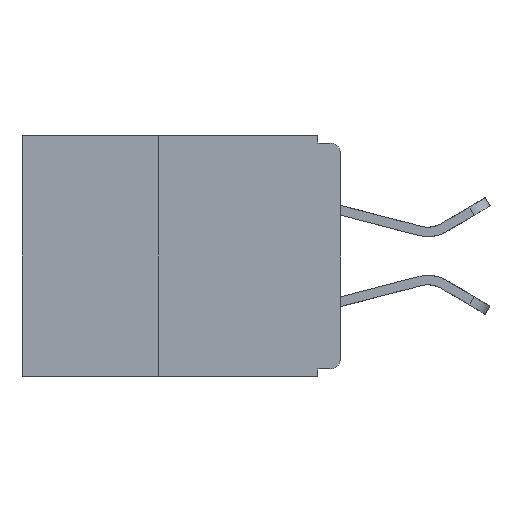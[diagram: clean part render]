
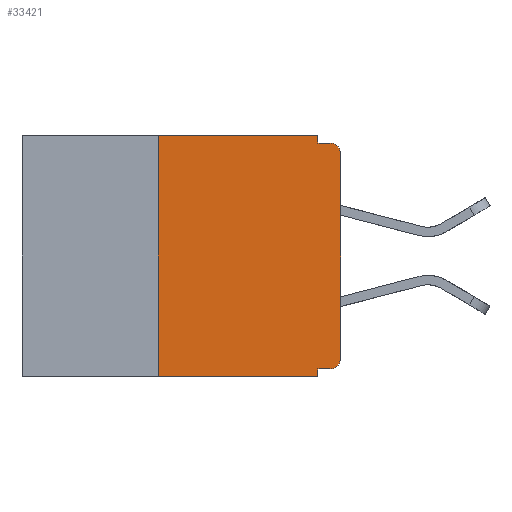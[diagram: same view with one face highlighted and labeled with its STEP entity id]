
A CAD part, left-side view. The second image highlights one B-rep face of the part: STEP entity #33421.
In plain terms, the highlighted planar face has unit normal (-1, 0, 0).
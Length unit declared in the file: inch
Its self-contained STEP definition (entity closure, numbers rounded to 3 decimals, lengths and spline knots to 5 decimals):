
#557 = DIRECTION ( 'NONE',  ( -1., 0., 0. ) ) ;
#912 = VECTOR ( 'NONE', #31816, 39.37008 ) ;
#1109 = DIRECTION ( 'NONE',  ( 0., 0., -1. ) ) ;
#1717 = CARTESIAN_POINT ( 'NONE',  ( 0., 0.031, -0.33 ) ) ;
#2532 = CARTESIAN_POINT ( 'NONE',  ( 0., 0.031, 0. ) ) ;
#2622 = EDGE_CURVE ( 'NONE', #32373, #4309, #14966, .T. ) ;
#2634 = CARTESIAN_POINT ( 'NONE',  ( 0., 0., -0.305 ) ) ;
#3227 = ORIENTED_EDGE ( 'NONE', *, *, #11046, .F. ) ;
#3566 = DIRECTION ( 'NONE',  ( -1., 0., 0. ) ) ;
#3796 = VERTEX_POINT ( 'NONE', #2532 ) ;
#4309 = VERTEX_POINT ( 'NONE', #1717 ) ;
#6083 = DIRECTION ( 'NONE',  ( 0., 0., -1. ) ) ;
#6546 = VERTEX_POINT ( 'NONE', #23697 ) ;
#7873 = VERTEX_POINT ( 'NONE', #2634 ) ;
#8239 = CARTESIAN_POINT ( 'NONE',  ( 0., 0., 0. ) ) ;
#9214 = DIRECTION ( 'NONE',  ( 1., 0., 0. ) ) ;
#9458 = AXIS2_PLACEMENT_3D ( 'NONE', #19245, #3566, #21910 ) ;
#9870 = LINE ( 'NONE', #29517, #32425 ) ;
#10485 = DIRECTION ( 'NONE',  ( 0., 0., 1. ) ) ;
#11046 = EDGE_CURVE ( 'NONE', #21604, #4309, #32266, .T. ) ;
#11399 = CARTESIAN_POINT ( 'NONE',  ( 0., 0.031, -0.33 ) ) ;
#11417 = CARTESIAN_POINT ( 'NONE',  ( 0., 0.031, -0.32 ) ) ;
#11556 = CARTESIAN_POINT ( 'NONE',  ( 0., 0.437, 0. ) ) ;
#11889 = ORIENTED_EDGE ( 'NONE', *, *, #33866, .F. ) ;
#12081 = AXIS2_PLACEMENT_3D ( 'NONE', #16334, #557, #18958 ) ;
#12883 = VERTEX_POINT ( 'NONE', #18671 ) ;
#13077 = CARTESIAN_POINT ( 'NONE',  ( 0., 0., -0.01 ) ) ;
#13196 = DIRECTION ( 'NONE',  ( 0., -1., 0. ) ) ;
#14277 = DIRECTION ( 'NONE',  ( 0., -1., 0. ) ) ;
#14318 = ORIENTED_EDGE ( 'NONE', *, *, #22124, .T. ) ;
#14966 = LINE ( 'NONE', #25424, #912 ) ;
#15114 = ORIENTED_EDGE ( 'NONE', *, *, #20731, .F. ) ;
#15219 = VERTEX_POINT ( 'NONE', #23155 ) ;
#16013 = VECTOR ( 'NONE', #14277, 39.37008 ) ;
#16090 = DIRECTION ( 'NONE',  ( 0., 0., 1. ) ) ;
#16334 = CARTESIAN_POINT ( 'NONE',  ( 0., 0.015, -0.025 ) ) ;
#16618 = CARTESIAN_POINT ( 'NONE',  ( 0., 0.25, 0. ) ) ;
#16709 = ORIENTED_EDGE ( 'NONE', *, *, #23192, .F. ) ;
#16944 = PLANE ( 'NONE',  #30615 ) ;
#17109 = VERTEX_POINT ( 'NONE', #16618 ) ;
#17539 = ORIENTED_EDGE ( 'NONE', *, *, #25066, .F. ) ;
#18671 = CARTESIAN_POINT ( 'NONE',  ( 0., 0.015, -0.01 ) ) ;
#18958 = DIRECTION ( 'NONE',  ( 0., 0., -1. ) ) ;
#19245 = CARTESIAN_POINT ( 'NONE',  ( 0., 0.015, -0.305 ) ) ;
#19425 = VECTOR ( 'NONE', #1109, 39.37008 ) ;
#20249 = LINE ( 'NONE', #32608, #19425 ) ;
#20731 = EDGE_CURVE ( 'NONE', #27944, #12883, #32709, .T. ) ;
#20837 = EDGE_CURVE ( 'NONE', #15219, #12883, #22433, .T. ) ;
#21604 = VERTEX_POINT ( 'NONE', #11417 ) ;
#21910 = DIRECTION ( 'NONE',  ( 0., 0., -1. ) ) ;
#22124 = EDGE_CURVE ( 'NONE', #6546, #7873, #25335, .T. ) ;
#22433 = CIRCLE ( 'NONE', #12081, 0.015 ) ;
#23030 = CARTESIAN_POINT ( 'NONE',  ( 0., 0.25, -0.33 ) ) ;
#23155 = CARTESIAN_POINT ( 'NONE',  ( 0., 0., -0.025 ) ) ;
#23192 = EDGE_CURVE ( 'NONE', #3796, #27944, #20249, .T. ) ;
#23697 = CARTESIAN_POINT ( 'NONE',  ( 0., 0.015, -0.32 ) ) ;
#24935 = CARTESIAN_POINT ( 'NONE',  ( 0., 0.437, 0. ) ) ;
#25066 = EDGE_CURVE ( 'NONE', #17109, #3796, #30035, .T. ) ;
#25335 = CIRCLE ( 'NONE', #9458, 0.015 ) ;
#25423 = ORIENTED_EDGE ( 'NONE', *, *, #33110, .F. ) ;
#25424 = CARTESIAN_POINT ( 'NONE',  ( 0., 0.437, -0.33 ) ) ;
#25801 = VECTOR ( 'NONE', #13196, 39.37008 ) ;
#26629 = ORIENTED_EDGE ( 'NONE', *, *, #29380, .T. ) ;
#27131 = LINE ( 'NONE', #31520, #32418 ) ;
#27588 = DIRECTION ( 'NONE',  ( 0., 0., -1. ) ) ;
#27944 = VERTEX_POINT ( 'NONE', #29426 ) ;
#28269 = ORIENTED_EDGE ( 'NONE', *, *, #20837, .T. ) ;
#29380 = EDGE_CURVE ( 'NONE', #7873, #15219, #33612, .T. ) ;
#29426 = CARTESIAN_POINT ( 'NONE',  ( 0., 0.031, -0.01 ) ) ;
#29517 = CARTESIAN_POINT ( 'NONE',  ( 0., 0., -0.32 ) ) ;
#29577 = FACE_OUTER_BOUND ( 'NONE', #33603, .T. ) ;
#30035 = LINE ( 'NONE', #11556, #16013 ) ;
#30615 = AXIS2_PLACEMENT_3D ( 'NONE', #24935, #9214, #27588 ) ;
#31486 = VECTOR ( 'NONE', #6083, 39.37008 ) ;
#31520 = CARTESIAN_POINT ( 'NONE',  ( 0., 0.25, -0.33 ) ) ;
#31816 = DIRECTION ( 'NONE',  ( 0., -1., 0. ) ) ;
#32112 = DIRECTION ( 'NONE',  ( 0., 1., 0. ) ) ;
#32266 = LINE ( 'NONE', #11399, #31486 ) ;
#32373 = VERTEX_POINT ( 'NONE', #23030 ) ;
#32418 = VECTOR ( 'NONE', #10485, 39.37008 ) ;
#32425 = VECTOR ( 'NONE', #32112, 39.37008 ) ;
#32608 = CARTESIAN_POINT ( 'NONE',  ( 0., 0.031, 0. ) ) ;
#32709 = LINE ( 'NONE', #13077, #25801 ) ;
#32831 = VECTOR ( 'NONE', #16090, 39.37008 ) ;
#33110 = EDGE_CURVE ( 'NONE', #32373, #17109, #27131, .T. ) ;
#33151 = ORIENTED_EDGE ( 'NONE', *, *, #2622, .T. ) ;
#33421 = ADVANCED_FACE ( 'NONE', ( #29577 ), #16944, .F. ) ;
#33603 = EDGE_LOOP ( 'NONE', ( #26629, #28269, #15114, #16709, #17539, #25423, #33151, #3227, #11889, #14318 ) ) ;
#33612 = LINE ( 'NONE', #8239, #32831 ) ;
#33866 = EDGE_CURVE ( 'NONE', #6546, #21604, #9870, .T. ) ;
